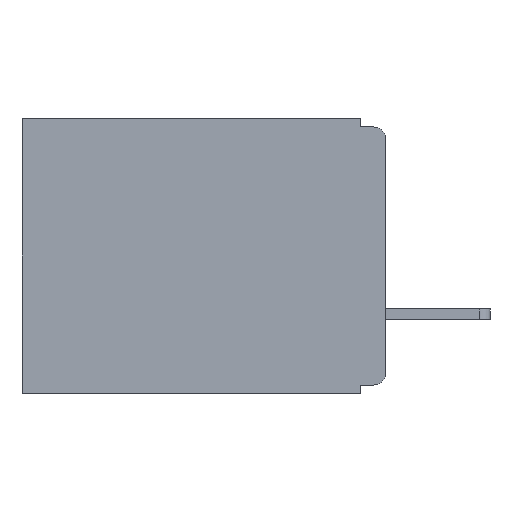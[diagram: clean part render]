
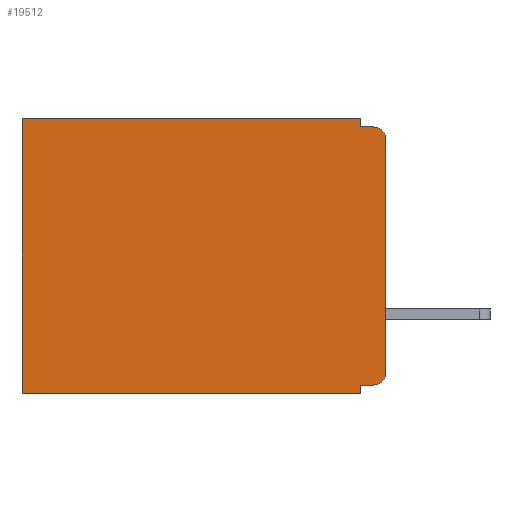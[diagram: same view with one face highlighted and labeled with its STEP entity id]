
A CAD part, left-side view. The second image highlights one B-rep face of the part: STEP entity #19512.
In plain terms, the highlighted planar face has unit normal (-1, 0, 0).
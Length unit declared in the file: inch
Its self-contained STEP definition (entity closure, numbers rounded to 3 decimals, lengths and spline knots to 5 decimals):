
#201 = DIRECTION ( 'NONE',  ( 0., 1., 0. ) ) ;
#1368 = LINE ( 'NONE', #10031, #14403 ) ;
#1688 = VECTOR ( 'NONE', #3645, 39.37008 ) ;
#3057 = VERTEX_POINT ( 'NONE', #14219 ) ;
#3645 = DIRECTION ( 'NONE',  ( 0., 0., -1. ) ) ;
#3749 = VECTOR ( 'NONE', #8008, 39.37008 ) ;
#4228 = DIRECTION ( 'NONE',  ( 0., -1., 0. ) ) ;
#4514 = CARTESIAN_POINT ( 'NONE',  ( 0.3, 0.031, -0.32 ) ) ;
#5364 = CARTESIAN_POINT ( 'NONE',  ( 0.3, 0., -0.32 ) ) ;
#5500 = CARTESIAN_POINT ( 'NONE',  ( 0.3, 0.031, -0.01 ) ) ;
#5754 = EDGE_CURVE ( 'NONE', #3057, #22931, #19374, .T. ) ;
#5765 = AXIS2_PLACEMENT_3D ( 'NONE', #11819, #6747, #24826 ) ;
#6653 = LINE ( 'NONE', #28905, #8296 ) ;
#6747 = DIRECTION ( 'NONE',  ( 1., 0., 0. ) ) ;
#6845 = CARTESIAN_POINT ( 'NONE',  ( 0.3, 0.031, -0.33 ) ) ;
#7170 = ORIENTED_EDGE ( 'NONE', *, *, #19292, .F. ) ;
#8008 = DIRECTION ( 'NONE',  ( 0., 1., 0. ) ) ;
#8173 = LINE ( 'NONE', #13173, #27939 ) ;
#8296 = VECTOR ( 'NONE', #26404, 39.37008 ) ;
#8659 = AXIS2_PLACEMENT_3D ( 'NONE', #26741, #28082, #33047 ) ;
#9587 = CARTESIAN_POINT ( 'NONE',  ( 0.3, 0.437, -0.33 ) ) ;
#9848 = LINE ( 'NONE', #5364, #3749 ) ;
#10031 = CARTESIAN_POINT ( 'NONE',  ( 0.3, 0., -0.33 ) ) ;
#10235 = VECTOR ( 'NONE', #32793, 39.37008 ) ;
#10436 = EDGE_CURVE ( 'NONE', #22638, #15661, #1368, .T. ) ;
#10849 = DIRECTION ( 'NONE',  ( -1., 0., 0. ) ) ;
#11819 = CARTESIAN_POINT ( 'NONE',  ( 0.3, 0., -0.33 ) ) ;
#12325 = ORIENTED_EDGE ( 'NONE', *, *, #31718, .F. ) ;
#12528 = EDGE_CURVE ( 'NONE', #3057, #14865, #29231, .T. ) ;
#12608 = DIRECTION ( 'NONE',  ( 0., 1., 0. ) ) ;
#12847 = VERTEX_POINT ( 'NONE', #14267 ) ;
#13173 = CARTESIAN_POINT ( 'NONE',  ( 0.3, 0., 0. ) ) ;
#13607 = EDGE_CURVE ( 'NONE', #23972, #22931, #29354, .T. ) ;
#14219 = CARTESIAN_POINT ( 'NONE',  ( 0.3, 0., -0.025 ) ) ;
#14267 = CARTESIAN_POINT ( 'NONE',  ( 0.3, 0.031, 0. ) ) ;
#14403 = VECTOR ( 'NONE', #12608, 39.37008 ) ;
#14823 = VECTOR ( 'NONE', #4228, 39.37008 ) ;
#14865 = VERTEX_POINT ( 'NONE', #25174 ) ;
#15639 = EDGE_CURVE ( 'NONE', #25248, #15661, #24774, .T. ) ;
#15661 = VERTEX_POINT ( 'NONE', #22570 ) ;
#16574 = CARTESIAN_POINT ( 'NONE',  ( 0.3, 0., -0.33 ) ) ;
#17051 = PLANE ( 'NONE',  #5765 ) ;
#17537 = EDGE_CURVE ( 'NONE', #32954, #22638, #25016, .T. ) ;
#17984 = CARTESIAN_POINT ( 'NONE',  ( 0.3, 0.015, -0.32 ) ) ;
#18989 = ORIENTED_EDGE ( 'NONE', *, *, #12528, .F. ) ;
#19127 = VERTEX_POINT ( 'NONE', #17984 ) ;
#19292 = EDGE_CURVE ( 'NONE', #12847, #23972, #6653, .T. ) ;
#19374 = CIRCLE ( 'NONE', #8659, 0.015 ) ;
#19512 = ADVANCED_FACE ( 'NONE', ( #27302 ), #17051, .F. ) ;
#21727 = EDGE_CURVE ( 'NONE', #19127, #14865, #23899, .T. ) ;
#22220 = ORIENTED_EDGE ( 'NONE', *, *, #32576, .T. ) ;
#22570 = CARTESIAN_POINT ( 'NONE',  ( 0.3, 0.437, -0.33 ) ) ;
#22638 = VERTEX_POINT ( 'NONE', #32867 ) ;
#22931 = VERTEX_POINT ( 'NONE', #29165 ) ;
#23417 = VECTOR ( 'NONE', #25023, 39.37008 ) ;
#23655 = ORIENTED_EDGE ( 'NONE', *, *, #21727, .T. ) ;
#23899 = CIRCLE ( 'NONE', #32415, 0.015 ) ;
#23972 = VERTEX_POINT ( 'NONE', #5500 ) ;
#24774 = LINE ( 'NONE', #9587, #10235 ) ;
#24826 = DIRECTION ( 'NONE',  ( 0., 0., -1. ) ) ;
#25003 = ORIENTED_EDGE ( 'NONE', *, *, #5754, .T. ) ;
#25016 = LINE ( 'NONE', #6845, #23417 ) ;
#25023 = DIRECTION ( 'NONE',  ( 0., 0., -1. ) ) ;
#25174 = CARTESIAN_POINT ( 'NONE',  ( 0.3, 0., -0.305 ) ) ;
#25222 = ORIENTED_EDGE ( 'NONE', *, *, #13607, .F. ) ;
#25248 = VERTEX_POINT ( 'NONE', #29486 ) ;
#26309 = CARTESIAN_POINT ( 'NONE',  ( 0.3, 0.015, -0.305 ) ) ;
#26404 = DIRECTION ( 'NONE',  ( 0., 0., -1. ) ) ;
#26741 = CARTESIAN_POINT ( 'NONE',  ( 0.3, 0.015, -0.025 ) ) ;
#27302 = FACE_OUTER_BOUND ( 'NONE', #27834, .T. ) ;
#27834 = EDGE_LOOP ( 'NONE', ( #18989, #25003, #25222, #7170, #22220, #28073, #29564, #32905, #12325, #23655 ) ) ;
#27939 = VECTOR ( 'NONE', #201, 39.37008 ) ;
#28073 = ORIENTED_EDGE ( 'NONE', *, *, #15639, .T. ) ;
#28082 = DIRECTION ( 'NONE',  ( -1., 0., 0. ) ) ;
#28905 = CARTESIAN_POINT ( 'NONE',  ( 0.3, 0.031, 0. ) ) ;
#28924 = DIRECTION ( 'NONE',  ( 0., 0., -1. ) ) ;
#29165 = CARTESIAN_POINT ( 'NONE',  ( 0.3, 0.015, -0.01 ) ) ;
#29231 = LINE ( 'NONE', #16574, #1688 ) ;
#29354 = LINE ( 'NONE', #32679, #14823 ) ;
#29486 = CARTESIAN_POINT ( 'NONE',  ( 0.3, 0.437, 0. ) ) ;
#29564 = ORIENTED_EDGE ( 'NONE', *, *, #10436, .F. ) ;
#31718 = EDGE_CURVE ( 'NONE', #19127, #32954, #9848, .T. ) ;
#32415 = AXIS2_PLACEMENT_3D ( 'NONE', #26309, #10849, #28924 ) ;
#32576 = EDGE_CURVE ( 'NONE', #12847, #25248, #8173, .T. ) ;
#32679 = CARTESIAN_POINT ( 'NONE',  ( 0.3, 0., -0.01 ) ) ;
#32793 = DIRECTION ( 'NONE',  ( 0., 0., -1. ) ) ;
#32867 = CARTESIAN_POINT ( 'NONE',  ( 0.3, 0.031, -0.33 ) ) ;
#32905 = ORIENTED_EDGE ( 'NONE', *, *, #17537, .F. ) ;
#32954 = VERTEX_POINT ( 'NONE', #4514 ) ;
#33047 = DIRECTION ( 'NONE',  ( 0., 0., -1. ) ) ;
